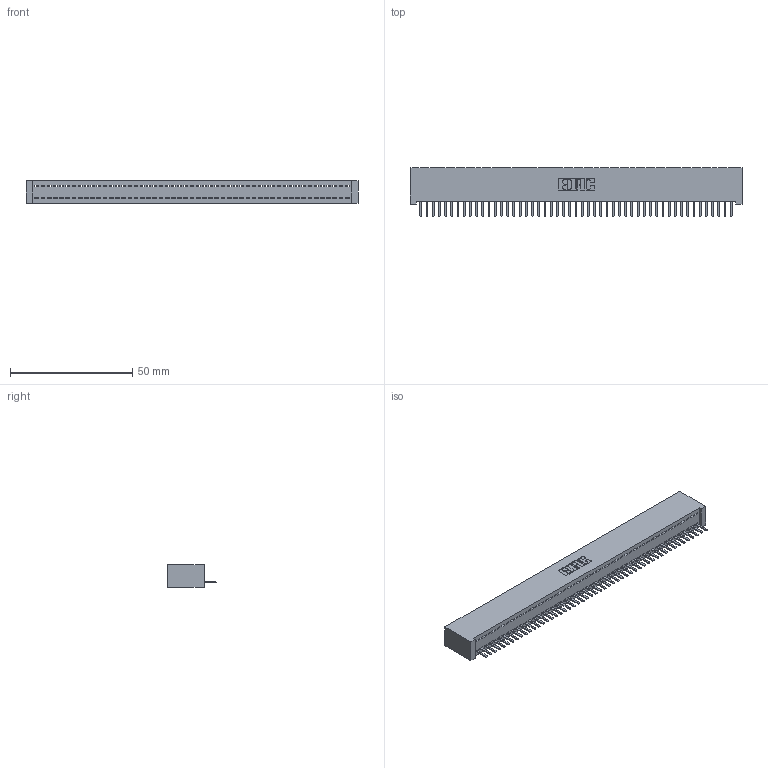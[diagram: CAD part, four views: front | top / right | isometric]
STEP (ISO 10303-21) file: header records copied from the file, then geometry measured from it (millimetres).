
FILE_DESCRIPTION (( 'STEP AP203' ), '1' );
FILE_NAME ('342-051-520-101.STEP', '2018-08-12T20:40:11', ( '' ), ( '' ), 'SwSTEP 2.0', 'SolidWorks 2016', '' );
FILE_SCHEMA (( 'CONFIG_CONTROL_DESIGN' ));
Length unit declared in the file: inch
Products named in the file (3): 345-292-001_345-293-120; 342-051-520-101; 342 Part_Lugless
Assembly tree (52 placements, depth 2):
  342-051-520-101
    342 Part_Lugless
    345-292-001_345-293-120  x51
Bounding box: 135.79 x 20.02 x 9.4 mm (x, y, z)
Volume: 12201.3 mm3; surface area: 17939.3 mm2
Topology: 52 solids, 52 shells, 3264 faces, 9659 edges, 6302 vertices
Faces by surface type: plane 2306, cylinder 958
Entity records: 29719 total; most frequent: CARTESIAN_POINT 5143, ORIENTED_EDGE 5118, DIRECTION 4301, EDGE_CURVE 2559, LINE 2435, VECTOR 2435, VERTEX_POINT 1702, AXIS2_PLACEMENT_3D 933
